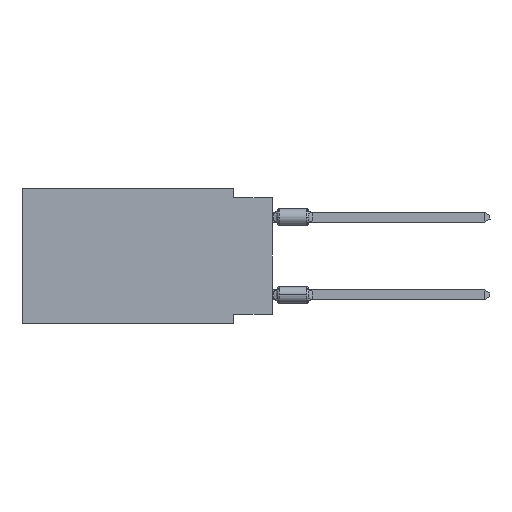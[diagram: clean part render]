
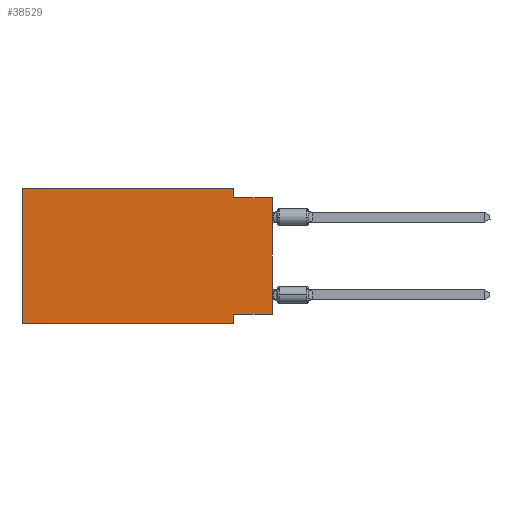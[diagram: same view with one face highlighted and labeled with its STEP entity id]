
A CAD part, left-side view. The second image highlights one B-rep face of the part: STEP entity #38529.
In plain terms, the highlighted planar face has unit normal (-1, 0, 0).
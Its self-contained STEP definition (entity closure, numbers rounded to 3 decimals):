
#2178 = CARTESIAN_POINT ( 'NONE',  ( 0., 16.383, 0. ) ) ;
#2716 = ORIENTED_EDGE ( 'NONE', *, *, #38111, .F. ) ;
#2992 = VECTOR ( 'NONE', #12945, 1000. ) ;
#3030 = EDGE_CURVE ( 'NONE', #13277, #31827, #56356, .T. ) ;
#4695 = ORIENTED_EDGE ( 'NONE', *, *, #3030, .F. ) ;
#6998 = CARTESIAN_POINT ( 'NONE',  ( 0., 16.383, -8.89 ) ) ;
#7907 = CARTESIAN_POINT ( 'NONE',  ( 0., 0., -0.635 ) ) ;
#7994 = DIRECTION ( 'NONE',  ( 0., -1., 0. ) ) ;
#8871 = CARTESIAN_POINT ( 'NONE',  ( 0., 2.54, 0. ) ) ;
#9397 = EDGE_LOOP ( 'NONE', ( #39936, #2716, #63628, #64737, #58408, #15302, #38629, #4695 ) ) ;
#9894 = EDGE_CURVE ( 'NONE', #13277, #23670, #35260, .T. ) ;
#10085 = CARTESIAN_POINT ( 'NONE',  ( 0., 16.383, 0. ) ) ;
#12945 = DIRECTION ( 'NONE',  ( 0., 1., 0. ) ) ;
#13277 = VERTEX_POINT ( 'NONE', #52449 ) ;
#14531 = EDGE_CURVE ( 'NONE', #31827, #60819, #16648, .T. ) ;
#15302 = ORIENTED_EDGE ( 'NONE', *, *, #50740, .T. ) ;
#16648 = LINE ( 'NONE', #67673, #29743 ) ;
#17131 = CARTESIAN_POINT ( 'NONE',  ( 0., 2.54, 0. ) ) ;
#18218 = PLANE ( 'NONE',  #69727 ) ;
#18574 = DIRECTION ( 'NONE',  ( 0., 0., -1. ) ) ;
#18804 = DIRECTION ( 'NONE',  ( 0., 0., 1. ) ) ;
#19584 = EDGE_CURVE ( 'NONE', #52691, #67707, #66232, .T. ) ;
#19659 = DIRECTION ( 'NONE',  ( 1., 0., 0. ) ) ;
#21545 = DIRECTION ( 'NONE',  ( 0., 0., -1. ) ) ;
#23670 = VERTEX_POINT ( 'NONE', #45714 ) ;
#27620 = DIRECTION ( 'NONE',  ( 0., 0., -1. ) ) ;
#29249 = DIRECTION ( 'NONE',  ( 0., -1., 0. ) ) ;
#29743 = VECTOR ( 'NONE', #27620, 1000. ) ;
#30518 = VECTOR ( 'NONE', #18804, 1000. ) ;
#31827 = VERTEX_POINT ( 'NONE', #50286 ) ;
#32512 = LINE ( 'NONE', #17131, #43548 ) ;
#33087 = DIRECTION ( 'NONE',  ( 0., 0., 1. ) ) ;
#35260 = LINE ( 'NONE', #36695, #30518 ) ;
#35733 = CARTESIAN_POINT ( 'NONE',  ( 0., 16.383, 0. ) ) ;
#36695 = CARTESIAN_POINT ( 'NONE',  ( 0., 0., 0. ) ) ;
#37247 = CARTESIAN_POINT ( 'NONE',  ( 0., 2.54, -0.635 ) ) ;
#38111 = EDGE_CURVE ( 'NONE', #70244, #23670, #47667, .T. ) ;
#38529 = ADVANCED_FACE ( 'NONE', ( #52498 ), #18218, .F. ) ;
#38629 = ORIENTED_EDGE ( 'NONE', *, *, #14531, .F. ) ;
#39936 = ORIENTED_EDGE ( 'NONE', *, *, #9894, .T. ) ;
#41215 = VECTOR ( 'NONE', #7994, 1000. ) ;
#43548 = VECTOR ( 'NONE', #21545, 1000. ) ;
#44373 = CARTESIAN_POINT ( 'NONE',  ( 0., 16.383, 0. ) ) ;
#44571 = CARTESIAN_POINT ( 'NONE',  ( 0., 2.54, -8.89 ) ) ;
#45714 = CARTESIAN_POINT ( 'NONE',  ( 0., 0., -0.635 ) ) ;
#47292 = DIRECTION ( 'NONE',  ( 0., -1., 0. ) ) ;
#47667 = LINE ( 'NONE', #7907, #68549 ) ;
#50286 = CARTESIAN_POINT ( 'NONE',  ( 0., 2.54, -8.255 ) ) ;
#50740 = EDGE_CURVE ( 'NONE', #52691, #60819, #62771, .T. ) ;
#52449 = CARTESIAN_POINT ( 'NONE',  ( 0., 0., -8.255 ) ) ;
#52498 = FACE_OUTER_BOUND ( 'NONE', #9397, .T. ) ;
#52559 = CARTESIAN_POINT ( 'NONE',  ( 0., 16.383, -8.89 ) ) ;
#52691 = VERTEX_POINT ( 'NONE', #52559 ) ;
#55672 = EDGE_CURVE ( 'NONE', #56344, #70244, #32512, .T. ) ;
#55974 = EDGE_CURVE ( 'NONE', #67707, #56344, #57937, .T. ) ;
#56344 = VERTEX_POINT ( 'NONE', #8871 ) ;
#56356 = LINE ( 'NONE', #57430, #2992 ) ;
#57430 = CARTESIAN_POINT ( 'NONE',  ( 0., 0., -8.255 ) ) ;
#57937 = LINE ( 'NONE', #35733, #41215 ) ;
#58408 = ORIENTED_EDGE ( 'NONE', *, *, #19584, .F. ) ;
#60497 = VECTOR ( 'NONE', #33087, 1000. ) ;
#60819 = VERTEX_POINT ( 'NONE', #44571 ) ;
#62771 = LINE ( 'NONE', #6998, #65041 ) ;
#63628 = ORIENTED_EDGE ( 'NONE', *, *, #55672, .F. ) ;
#64737 = ORIENTED_EDGE ( 'NONE', *, *, #55974, .F. ) ;
#65041 = VECTOR ( 'NONE', #29249, 1000. ) ;
#66232 = LINE ( 'NONE', #44373, #60497 ) ;
#67673 = CARTESIAN_POINT ( 'NONE',  ( 0., 2.54, -8.89 ) ) ;
#67707 = VERTEX_POINT ( 'NONE', #10085 ) ;
#68549 = VECTOR ( 'NONE', #47292, 1000. ) ;
#69727 = AXIS2_PLACEMENT_3D ( 'NONE', #2178, #19659, #18574 ) ;
#70244 = VERTEX_POINT ( 'NONE', #37247 ) ;
